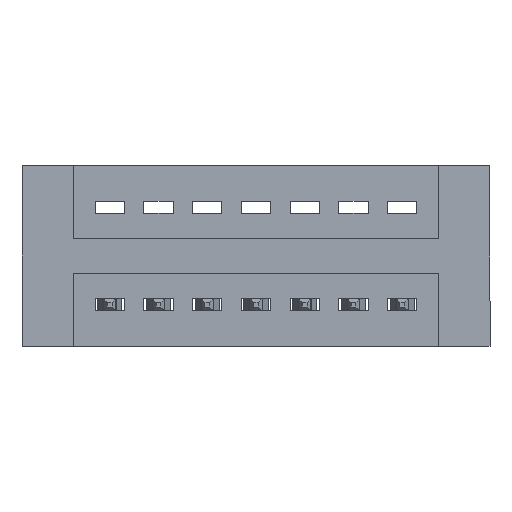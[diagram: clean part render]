
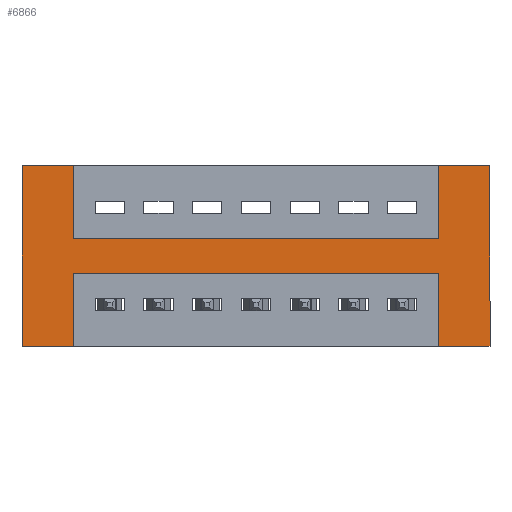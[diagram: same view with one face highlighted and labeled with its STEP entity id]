
A CAD part, front view. The second image highlights one B-rep face of the part: STEP entity #6866.
In plain terms, the highlighted planar face has unit normal (0, -1, 0).
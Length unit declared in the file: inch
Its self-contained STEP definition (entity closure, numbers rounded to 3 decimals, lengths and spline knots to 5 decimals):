
#1 = CARTESIAN_POINT ( 'NONE',  ( 1.2475, 0., 0. ) ) ;
#33 = CARTESIAN_POINT ( 'NONE',  ( 0.2875, 0., 0. ) ) ;
#109 = ORIENTED_EDGE ( 'NONE', *, *, #2206, .F. ) ;
#111 = CARTESIAN_POINT ( 'NONE',  ( 1.1425, 0., -0.37 ) ) ;
#210 = CARTESIAN_POINT ( 'NONE',  ( 0.3925, 0., -0.37 ) ) ;
#273 = CARTESIAN_POINT ( 'NONE',  ( 0.3925, 0., 0. ) ) ;
#347 = LINE ( 'NONE', #3325, #9603 ) ;
#380 = CARTESIAN_POINT ( 'NONE',  ( 0.3925, 0., -0.22 ) ) ;
#419 = CARTESIAN_POINT ( 'NONE',  ( 1.1425, 0., -0.22 ) ) ;
#525 = LINE ( 'NONE', #6931, #1331 ) ;
#538 = ORIENTED_EDGE ( 'NONE', *, *, #1375, .F. ) ;
#593 = ORIENTED_EDGE ( 'NONE', *, *, #1613, .F. ) ;
#743 = LINE ( 'NONE', #5104, #2633 ) ;
#746 = DIRECTION ( 'NONE',  ( 0., 0., -1. ) ) ;
#885 = VERTEX_POINT ( 'NONE', #6506 ) ;
#895 = VERTEX_POINT ( 'NONE', #5798 ) ;
#1237 = VECTOR ( 'NONE', #9662, 39.37008 ) ;
#1267 = EDGE_CURVE ( 'NONE', #895, #8863, #3678, .T. ) ;
#1331 = VECTOR ( 'NONE', #3264, 39.37008 ) ;
#1351 = CARTESIAN_POINT ( 'NONE',  ( 0.2875, 0., -0.37 ) ) ;
#1375 = EDGE_CURVE ( 'NONE', #6837, #6989, #2392, .T. ) ;
#1613 = EDGE_CURVE ( 'NONE', #4385, #8863, #8140, .T. ) ;
#1765 = EDGE_CURVE ( 'NONE', #9186, #9230, #8461, .T. ) ;
#2031 = DIRECTION ( 'NONE',  ( -1., 0., 0. ) ) ;
#2076 = ORIENTED_EDGE ( 'NONE', *, *, #3658, .F. ) ;
#2112 = VECTOR ( 'NONE', #9086, 39.37008 ) ;
#2206 = EDGE_CURVE ( 'NONE', #4655, #4385, #3191, .T. ) ;
#2294 = CARTESIAN_POINT ( 'NONE',  ( 0., 0., -0.37 ) ) ;
#2352 = DIRECTION ( 'NONE',  ( 0., 0., 1. ) ) ;
#2392 = LINE ( 'NONE', #111, #4141 ) ;
#2393 = ORIENTED_EDGE ( 'NONE', *, *, #1765, .F. ) ;
#2445 = DIRECTION ( 'NONE',  ( 0., 0., -1. ) ) ;
#2633 = VECTOR ( 'NONE', #5740, 39.37008 ) ;
#2980 = VECTOR ( 'NONE', #746, 39.37008 ) ;
#3050 = EDGE_LOOP ( 'NONE', ( #9549, #9171, #7798, #2076, #2393, #9020, #3210, #593, #109, #4792, #538, #3745 ) ) ;
#3191 = LINE ( 'NONE', #5592, #9049 ) ;
#3210 = ORIENTED_EDGE ( 'NONE', *, *, #1267, .T. ) ;
#3264 = DIRECTION ( 'NONE',  ( 1., 0., 0. ) ) ;
#3312 = EDGE_CURVE ( 'NONE', #6989, #4655, #4914, .T. ) ;
#3325 = CARTESIAN_POINT ( 'NONE',  ( 0.3925, 0., -0.15 ) ) ;
#3572 = VECTOR ( 'NONE', #3940, 39.37008 ) ;
#3658 = EDGE_CURVE ( 'NONE', #9230, #9651, #347, .T. ) ;
#3665 = DIRECTION ( 'NONE',  ( 0., 0., 1. ) ) ;
#3678 = LINE ( 'NONE', #33, #2980 ) ;
#3745 = ORIENTED_EDGE ( 'NONE', *, *, #9574, .F. ) ;
#3806 = FACE_OUTER_BOUND ( 'NONE', #3050, .T. ) ;
#3940 = DIRECTION ( 'NONE',  ( 0., 0., 1. ) ) ;
#4000 = LINE ( 'NONE', #1, #8892 ) ;
#4141 = VECTOR ( 'NONE', #2352, 39.37008 ) ;
#4385 = VERTEX_POINT ( 'NONE', #210 ) ;
#4524 = AXIS2_PLACEMENT_3D ( 'NONE', #4731, #8496, #2445 ) ;
#4628 = PLANE ( 'NONE',  #4524 ) ;
#4655 = VERTEX_POINT ( 'NONE', #5293 ) ;
#4731 = CARTESIAN_POINT ( 'NONE',  ( 0., 0., -0.37 ) ) ;
#4792 = ORIENTED_EDGE ( 'NONE', *, *, #3312, .F. ) ;
#4914 = LINE ( 'NONE', #380, #5838 ) ;
#4950 = DIRECTION ( 'NONE',  ( 0., 0., -1. ) ) ;
#5104 = CARTESIAN_POINT ( 'NONE',  ( 0., 0., 0. ) ) ;
#5293 = CARTESIAN_POINT ( 'NONE',  ( 0.3925, 0., -0.22 ) ) ;
#5417 = CARTESIAN_POINT ( 'NONE',  ( 1.1425, 0., -0.37 ) ) ;
#5470 = CARTESIAN_POINT ( 'NONE',  ( 0.3925, 0., 0. ) ) ;
#5592 = CARTESIAN_POINT ( 'NONE',  ( 0.3925, 0., -0.37 ) ) ;
#5705 = CARTESIAN_POINT ( 'NONE',  ( 1.2475, 0., 0. ) ) ;
#5740 = DIRECTION ( 'NONE',  ( 1., 0., 0. ) ) ;
#5756 = VERTEX_POINT ( 'NONE', #5705 ) ;
#5798 = CARTESIAN_POINT ( 'NONE',  ( 0.2875, 0., 0. ) ) ;
#5838 = VECTOR ( 'NONE', #2031, 39.37008 ) ;
#6200 = CARTESIAN_POINT ( 'NONE',  ( 1.1425, 0., -0.15 ) ) ;
#6455 = VECTOR ( 'NONE', #7023, 39.37008 ) ;
#6506 = CARTESIAN_POINT ( 'NONE',  ( 1.1425, 0., 0. ) ) ;
#6698 = LINE ( 'NONE', #6747, #3572 ) ;
#6747 = CARTESIAN_POINT ( 'NONE',  ( 1.1425, 0., 0. ) ) ;
#6831 = EDGE_CURVE ( 'NONE', #895, #9186, #525, .T. ) ;
#6837 = VERTEX_POINT ( 'NONE', #5417 ) ;
#6866 = ADVANCED_FACE ( 'NONE', ( #3806 ), #4628, .T. ) ;
#6931 = CARTESIAN_POINT ( 'NONE',  ( 0., 0., 0. ) ) ;
#6989 = VERTEX_POINT ( 'NONE', #419 ) ;
#7023 = DIRECTION ( 'NONE',  ( 0., 0., -1. ) ) ;
#7711 = EDGE_CURVE ( 'NONE', #9299, #5756, #4000, .T. ) ;
#7798 = ORIENTED_EDGE ( 'NONE', *, *, #7858, .F. ) ;
#7858 = EDGE_CURVE ( 'NONE', #9651, #885, #6698, .T. ) ;
#7936 = DIRECTION ( 'NONE',  ( 1., 0., 0. ) ) ;
#8140 = LINE ( 'NONE', #8885, #1237 ) ;
#8290 = EDGE_CURVE ( 'NONE', #885, #5756, #743, .T. ) ;
#8461 = LINE ( 'NONE', #5470, #6455 ) ;
#8464 = CARTESIAN_POINT ( 'NONE',  ( 1.2475, 0., -0.37 ) ) ;
#8496 = DIRECTION ( 'NONE',  ( 0., -1., 0. ) ) ;
#8863 = VERTEX_POINT ( 'NONE', #1351 ) ;
#8885 = CARTESIAN_POINT ( 'NONE',  ( 0., 0., -0.37 ) ) ;
#8892 = VECTOR ( 'NONE', #3665, 39.37008 ) ;
#8919 = LINE ( 'NONE', #2294, #2112 ) ;
#9020 = ORIENTED_EDGE ( 'NONE', *, *, #6831, .F. ) ;
#9049 = VECTOR ( 'NONE', #4950, 39.37008 ) ;
#9086 = DIRECTION ( 'NONE',  ( -1., 0., 0. ) ) ;
#9171 = ORIENTED_EDGE ( 'NONE', *, *, #8290, .F. ) ;
#9186 = VERTEX_POINT ( 'NONE', #273 ) ;
#9219 = CARTESIAN_POINT ( 'NONE',  ( 0.3925, 0., -0.15 ) ) ;
#9230 = VERTEX_POINT ( 'NONE', #9219 ) ;
#9299 = VERTEX_POINT ( 'NONE', #8464 ) ;
#9549 = ORIENTED_EDGE ( 'NONE', *, *, #7711, .T. ) ;
#9574 = EDGE_CURVE ( 'NONE', #9299, #6837, #8919, .T. ) ;
#9603 = VECTOR ( 'NONE', #7936, 39.37008 ) ;
#9651 = VERTEX_POINT ( 'NONE', #6200 ) ;
#9662 = DIRECTION ( 'NONE',  ( -1., 0., 0. ) ) ;
